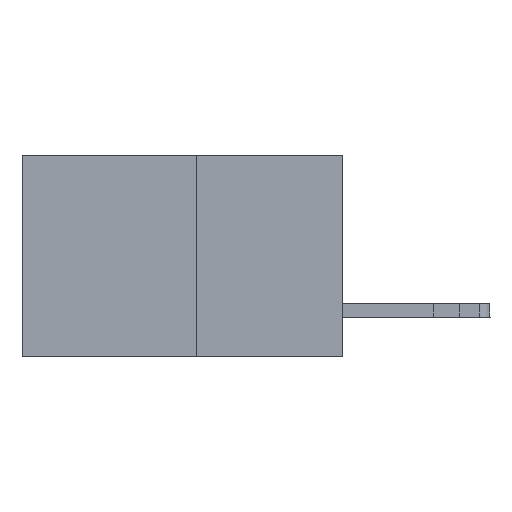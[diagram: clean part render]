
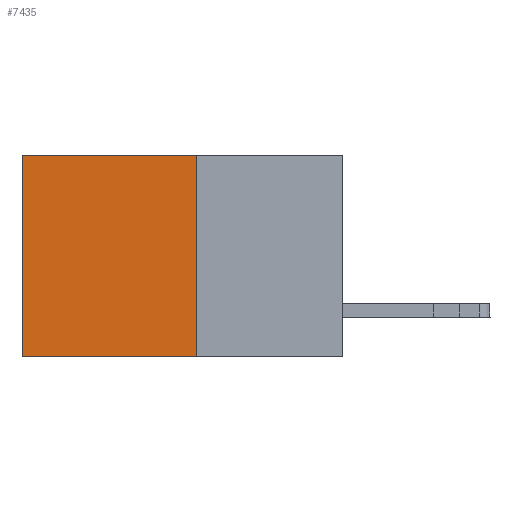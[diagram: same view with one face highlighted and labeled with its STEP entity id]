
A CAD part, left-side view. The second image highlights one B-rep face of the part: STEP entity #7435.
In plain terms, the highlighted planar face has unit normal (-1, 0, 0).
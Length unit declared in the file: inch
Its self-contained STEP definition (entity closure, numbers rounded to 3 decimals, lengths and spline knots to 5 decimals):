
#95 = DIRECTION ( 'NONE',  ( 1., 0., 0. ) ) ;
#271 = DIRECTION ( 'NONE',  ( 0., 0., -1. ) ) ;
#627 = CARTESIAN_POINT ( 'NONE',  ( 0.277, 0.27, -0.37 ) ) ;
#1248 = ORIENTED_EDGE ( 'NONE', *, *, #14682, .T. ) ;
#1883 = DIRECTION ( 'NONE',  ( 0., 1., 0. ) ) ;
#2213 = CARTESIAN_POINT ( 'NONE',  ( 0.277, 0.59, 0. ) ) ;
#3587 = EDGE_CURVE ( 'NONE', #5328, #10549, #10661, .T. ) ;
#4692 = ORIENTED_EDGE ( 'NONE', *, *, #13595, .T. ) ;
#4788 = VECTOR ( 'NONE', #11139, 39.37008 ) ;
#5220 = ORIENTED_EDGE ( 'NONE', *, *, #3587, .F. ) ;
#5328 = VERTEX_POINT ( 'NONE', #6115 ) ;
#5380 = CARTESIAN_POINT ( 'NONE',  ( 0.277, 0.27, 0. ) ) ;
#5873 = DIRECTION ( 'NONE',  ( 0., 0., -1. ) ) ;
#6115 = CARTESIAN_POINT ( 'NONE',  ( 0.277, 0.27, 0. ) ) ;
#6510 = LINE ( 'NONE', #15325, #7165 ) ;
#6787 = LINE ( 'NONE', #5380, #4788 ) ;
#7128 = AXIS2_PLACEMENT_3D ( 'NONE', #9946, #95, #5873 ) ;
#7165 = VECTOR ( 'NONE', #13908, 39.37008 ) ;
#7302 = PLANE ( 'NONE',  #7128 ) ;
#7435 = ADVANCED_FACE ( 'NONE', ( #8718 ), #7302, .F. ) ;
#7602 = EDGE_CURVE ( 'NONE', #10549, #16502, #14951, .T. ) ;
#8192 = CARTESIAN_POINT ( 'NONE',  ( 0.277, 0.59, -0.37 ) ) ;
#8718 = FACE_OUTER_BOUND ( 'NONE', #9306, .T. ) ;
#9122 = VERTEX_POINT ( 'NONE', #2213 ) ;
#9306 = EDGE_LOOP ( 'NONE', ( #1248, #16048, #5220, #4692 ) ) ;
#9946 = CARTESIAN_POINT ( 'NONE',  ( 0.277, 0.27, -0.37 ) ) ;
#10549 = VERTEX_POINT ( 'NONE', #627 ) ;
#10661 = LINE ( 'NONE', #11824, #13196 ) ;
#11139 = DIRECTION ( 'NONE',  ( 0., 1., 0. ) ) ;
#11824 = CARTESIAN_POINT ( 'NONE',  ( 0.277, 0.27, -0.37 ) ) ;
#13196 = VECTOR ( 'NONE', #271, 39.37008 ) ;
#13595 = EDGE_CURVE ( 'NONE', #5328, #9122, #6787, .T. ) ;
#13908 = DIRECTION ( 'NONE',  ( 0., 0., -1. ) ) ;
#14682 = EDGE_CURVE ( 'NONE', #9122, #16502, #6510, .T. ) ;
#14951 = LINE ( 'NONE', #17711, #18647 ) ;
#15325 = CARTESIAN_POINT ( 'NONE',  ( 0.277, 0.59, -0.37 ) ) ;
#16048 = ORIENTED_EDGE ( 'NONE', *, *, #7602, .F. ) ;
#16502 = VERTEX_POINT ( 'NONE', #8192 ) ;
#17711 = CARTESIAN_POINT ( 'NONE',  ( 0.277, 0.27, -0.37 ) ) ;
#18647 = VECTOR ( 'NONE', #1883, 39.37008 ) ;
